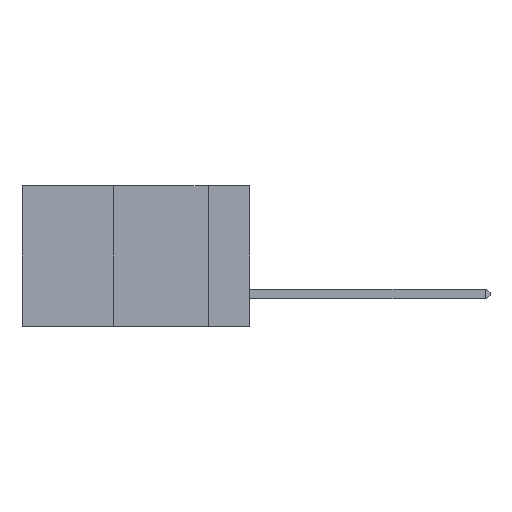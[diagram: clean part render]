
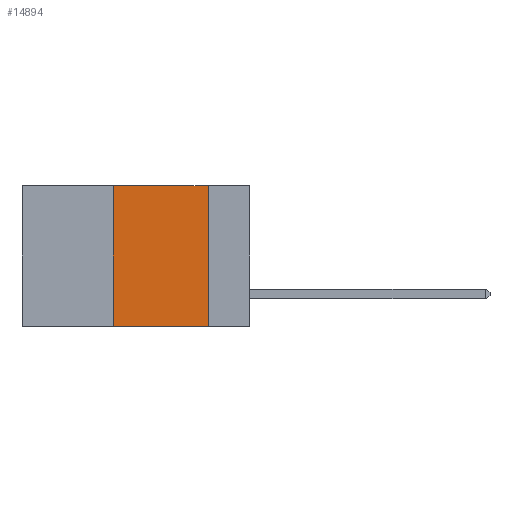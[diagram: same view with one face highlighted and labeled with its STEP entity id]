
A CAD part, left-side view. The second image highlights one B-rep face of the part: STEP entity #14894.
In plain terms, the highlighted planar face has unit normal (-1, 0, 0).
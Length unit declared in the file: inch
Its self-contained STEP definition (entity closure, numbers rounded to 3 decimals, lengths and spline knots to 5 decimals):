
#1446 = LINE ( 'NONE', #9198, #7525 ) ;
#2013 = CARTESIAN_POINT ( 'NONE',  ( 0., 0.6, 0. ) ) ;
#2477 = PLANE ( 'NONE',  #13110 ) ;
#2735 = ORIENTED_EDGE ( 'NONE', *, *, #15334, .F. ) ;
#3504 = EDGE_LOOP ( 'NONE', ( #15464, #2735, #12744, #15830 ) ) ;
#3953 = VERTEX_POINT ( 'NONE', #5011 ) ;
#4561 = VECTOR ( 'NONE', #9793, 39.37008 ) ;
#4764 = CARTESIAN_POINT ( 'NONE',  ( 0., 0.36, -0.37 ) ) ;
#4955 = LINE ( 'NONE', #8560, #4561 ) ;
#5011 = CARTESIAN_POINT ( 'NONE',  ( 0., 0.11, 0. ) ) ;
#5118 = LINE ( 'NONE', #2013, #8822 ) ;
#6110 = VECTOR ( 'NONE', #7225, 39.37008 ) ;
#6487 = LINE ( 'NONE', #12142, #6110 ) ;
#6532 = EDGE_CURVE ( 'NONE', #13982, #10228, #1446, .T. ) ;
#7225 = DIRECTION ( 'NONE',  ( 0., -1., 0. ) ) ;
#7272 = VERTEX_POINT ( 'NONE', #11966 ) ;
#7525 = VECTOR ( 'NONE', #10432, 39.37008 ) ;
#8202 = EDGE_CURVE ( 'NONE', #3953, #7272, #4955, .T. ) ;
#8560 = CARTESIAN_POINT ( 'NONE',  ( 0., 0.11, 0. ) ) ;
#8822 = VECTOR ( 'NONE', #14414, 39.37008 ) ;
#8842 = CARTESIAN_POINT ( 'NONE',  ( 0., 0.6, 0. ) ) ;
#9038 = EDGE_CURVE ( 'NONE', #13982, #7272, #6487, .T. ) ;
#9198 = CARTESIAN_POINT ( 'NONE',  ( 0., 0.36, 0. ) ) ;
#9793 = DIRECTION ( 'NONE',  ( 0., 0., -1. ) ) ;
#10228 = VERTEX_POINT ( 'NONE', #12996 ) ;
#10432 = DIRECTION ( 'NONE',  ( 0., 0., 1. ) ) ;
#11296 = DIRECTION ( 'NONE',  ( 0., 0., -1. ) ) ;
#11966 = CARTESIAN_POINT ( 'NONE',  ( 0., 0.11, -0.37 ) ) ;
#12142 = CARTESIAN_POINT ( 'NONE',  ( 0., 0.6, -0.37 ) ) ;
#12744 = ORIENTED_EDGE ( 'NONE', *, *, #6532, .F. ) ;
#12996 = CARTESIAN_POINT ( 'NONE',  ( 0., 0.36, 0. ) ) ;
#13110 = AXIS2_PLACEMENT_3D ( 'NONE', #8842, #13653, #11296 ) ;
#13653 = DIRECTION ( 'NONE',  ( 1., 0., 0. ) ) ;
#13982 = VERTEX_POINT ( 'NONE', #4764 ) ;
#14414 = DIRECTION ( 'NONE',  ( 0., -1., 0. ) ) ;
#14496 = FACE_OUTER_BOUND ( 'NONE', #3504, .T. ) ;
#14894 = ADVANCED_FACE ( 'NONE', ( #14496 ), #2477, .F. ) ;
#15334 = EDGE_CURVE ( 'NONE', #10228, #3953, #5118, .T. ) ;
#15464 = ORIENTED_EDGE ( 'NONE', *, *, #8202, .F. ) ;
#15830 = ORIENTED_EDGE ( 'NONE', *, *, #9038, .T. ) ;
